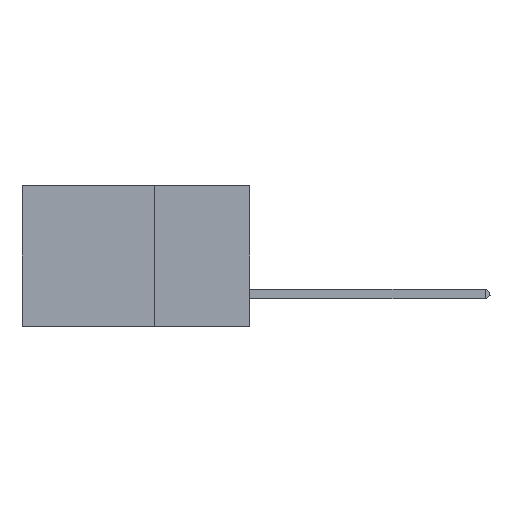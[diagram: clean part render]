
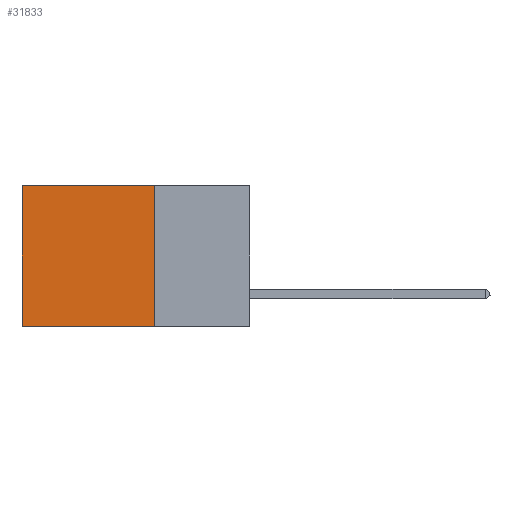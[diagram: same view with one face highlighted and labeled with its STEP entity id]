
A CAD part, left-side view. The second image highlights one B-rep face of the part: STEP entity #31833.
In plain terms, the highlighted planar face has unit normal (-1, 0, 0).
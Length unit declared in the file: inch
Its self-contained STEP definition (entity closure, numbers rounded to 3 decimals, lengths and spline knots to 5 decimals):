
#40 = CARTESIAN_POINT ( 'NONE',  ( 0.2875, 0.25, 0. ) ) ;
#1171 = ORIENTED_EDGE ( 'NONE', *, *, #19727, .F. ) ;
#3073 = VECTOR ( 'NONE', #21857, 39.37008 ) ;
#3154 = DIRECTION ( 'NONE',  ( 0., 0., -1. ) ) ;
#3672 = VECTOR ( 'NONE', #9959, 39.37008 ) ;
#4464 = VECTOR ( 'NONE', #9910, 39.37008 ) ;
#4666 = EDGE_LOOP ( 'NONE', ( #41842, #1171, #36160, #10017 ) ) ;
#4877 = CARTESIAN_POINT ( 'NONE',  ( 0.2875, 0.6, 0. ) ) ;
#5514 = LINE ( 'NONE', #16396, #4464 ) ;
#5772 = PLANE ( 'NONE',  #32767 ) ;
#6805 = LINE ( 'NONE', #29417, #3672 ) ;
#9910 = DIRECTION ( 'NONE',  ( 0., 1., 0. ) ) ;
#9959 = DIRECTION ( 'NONE',  ( 0., 0., -1. ) ) ;
#10017 = ORIENTED_EDGE ( 'NONE', *, *, #35290, .T. ) ;
#15300 = VERTEX_POINT ( 'NONE', #34291 ) ;
#16388 = FACE_OUTER_BOUND ( 'NONE', #4666, .T. ) ;
#16396 = CARTESIAN_POINT ( 'NONE',  ( 0.2875, 0.25, 0. ) ) ;
#18539 = DIRECTION ( 'NONE',  ( 0., 1., 0. ) ) ;
#19727 = EDGE_CURVE ( 'NONE', #41823, #29020, #20448, .T. ) ;
#20221 = CARTESIAN_POINT ( 'NONE',  ( 0.2875, 0.6, -0.37 ) ) ;
#20448 = LINE ( 'NONE', #31789, #38216 ) ;
#20474 = CARTESIAN_POINT ( 'NONE',  ( 0.2875, 0.25, -0.37 ) ) ;
#21857 = DIRECTION ( 'NONE',  ( 0., 0., -1. ) ) ;
#25169 = CARTESIAN_POINT ( 'NONE',  ( 0.2875, 0.25, 0. ) ) ;
#29020 = VERTEX_POINT ( 'NONE', #20221 ) ;
#29417 = CARTESIAN_POINT ( 'NONE',  ( 0.2875, 0.6, 0. ) ) ;
#31789 = CARTESIAN_POINT ( 'NONE',  ( 0.2875, 0.25, -0.37 ) ) ;
#31833 = ADVANCED_FACE ( 'NONE', ( #16388 ), #5772, .F. ) ;
#32767 = AXIS2_PLACEMENT_3D ( 'NONE', #40, #39554, #3154 ) ;
#33319 = VERTEX_POINT ( 'NONE', #4877 ) ;
#34291 = CARTESIAN_POINT ( 'NONE',  ( 0.2875, 0.25, 0. ) ) ;
#35290 = EDGE_CURVE ( 'NONE', #15300, #33319, #5514, .T. ) ;
#36160 = ORIENTED_EDGE ( 'NONE', *, *, #39615, .F. ) ;
#37563 = LINE ( 'NONE', #25169, #3073 ) ;
#38216 = VECTOR ( 'NONE', #18539, 39.37008 ) ;
#38401 = EDGE_CURVE ( 'NONE', #33319, #29020, #6805, .T. ) ;
#39554 = DIRECTION ( 'NONE',  ( 1., 0., 0. ) ) ;
#39615 = EDGE_CURVE ( 'NONE', #15300, #41823, #37563, .T. ) ;
#41823 = VERTEX_POINT ( 'NONE', #20474 ) ;
#41842 = ORIENTED_EDGE ( 'NONE', *, *, #38401, .T. ) ;
